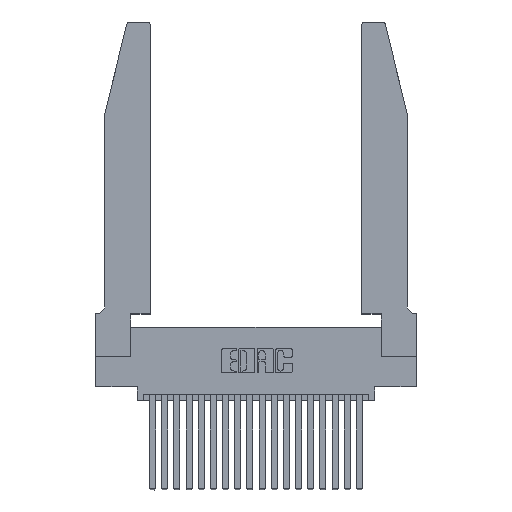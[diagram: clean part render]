
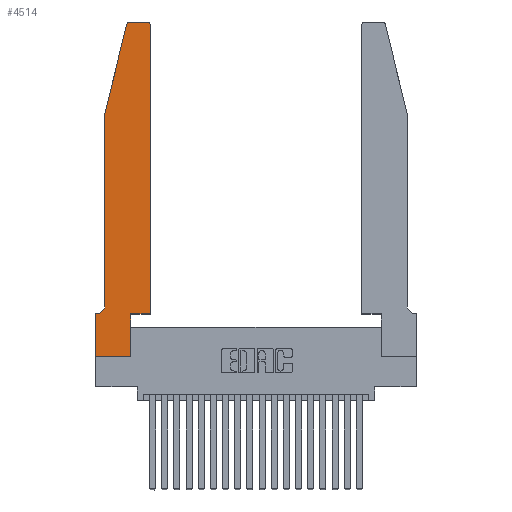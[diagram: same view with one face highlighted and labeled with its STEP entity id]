
A CAD part, top view. The second image highlights one B-rep face of the part: STEP entity #4514.
In plain terms, the highlighted planar face has unit normal (0, 0, 1).
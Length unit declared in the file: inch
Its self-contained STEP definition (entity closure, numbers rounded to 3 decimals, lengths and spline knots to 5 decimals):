
#236 = LINE ( 'NONE', #11558, #2390 ) ;
#587 = CARTESIAN_POINT ( 'NONE',  ( 0., 0., 0.37 ) ) ;
#653 = EDGE_CURVE ( 'NONE', #8122, #20150, #13571, .T. ) ;
#1013 = EDGE_CURVE ( 'NONE', #18267, #7652, #19644, .T. ) ;
#1073 = EDGE_CURVE ( 'NONE', #20150, #13080, #3122, .T. ) ;
#1366 = CIRCLE ( 'NONE', #17753, 0.03 ) ;
#1527 = DIRECTION ( 'NONE',  ( -1., 0., 0. ) ) ;
#1559 = DIRECTION ( 'NONE',  ( 1., 0., 0. ) ) ;
#1614 = VECTOR ( 'NONE', #1559, 39.37008 ) ;
#2044 = VECTOR ( 'NONE', #3336, 39.37008 ) ;
#2202 = AXIS2_PLACEMENT_3D ( 'NONE', #3374, #5071, #1527 ) ;
#2240 = CARTESIAN_POINT ( 'NONE',  ( 0., 0., 0.37 ) ) ;
#2390 = VECTOR ( 'NONE', #21987, 39.37008 ) ;
#2426 = LINE ( 'NONE', #10094, #1614 ) ;
#3022 = VERTEX_POINT ( 'NONE', #13504 ) ;
#3122 = LINE ( 'NONE', #21742, #2044 ) ;
#3255 = CARTESIAN_POINT ( 'NONE',  ( 0.4505, 0.35, 0.37 ) ) ;
#3336 = DIRECTION ( 'NONE',  ( -1., 0., 0. ) ) ;
#3374 = CARTESIAN_POINT ( 'NONE',  ( 0.0055, 0.42, 0.37 ) ) ;
#3446 = LINE ( 'NONE', #11900, #7200 ) ;
#3492 = LINE ( 'NONE', #2240, #19467 ) ;
#3637 = DIRECTION ( 'NONE',  ( 0., 0., 1. ) ) ;
#4107 = VERTEX_POINT ( 'NONE', #19464 ) ;
#4514 = ADVANCED_FACE ( 'NONE', ( #21670 ), #16902, .T. ) ;
#4571 = VERTEX_POINT ( 'NONE', #12188 ) ;
#4680 = DIRECTION ( 'NONE',  ( 1., 0., 0. ) ) ;
#4746 = CARTESIAN_POINT ( 'NONE',  ( 0.2605, 2.75, 0.37 ) ) ;
#5071 = DIRECTION ( 'NONE',  ( 0., 0., -1. ) ) ;
#5425 = DIRECTION ( 'NONE',  ( 1., 0., 0. ) ) ;
#5772 = VERTEX_POINT ( 'NONE', #10295 ) ;
#5898 = EDGE_CURVE ( 'NONE', #4107, #17096, #2426, .T. ) ;
#6042 = ORIENTED_EDGE ( 'NONE', *, *, #5898, .T. ) ;
#6260 = ORIENTED_EDGE ( 'NONE', *, *, #10911, .T. ) ;
#6274 = ORIENTED_EDGE ( 'NONE', *, *, #12861, .T. ) ;
#6558 = EDGE_CURVE ( 'NONE', #7302, #3022, #3446, .T. ) ;
#6589 = CARTESIAN_POINT ( 'NONE',  ( 0., 0.35, 0.37 ) ) ;
#7200 = VECTOR ( 'NONE', #20245, 39.37008 ) ;
#7202 = DIRECTION ( 'NONE',  ( 0., 0., 1. ) ) ;
#7302 = VERTEX_POINT ( 'NONE', #10898 ) ;
#7652 = VERTEX_POINT ( 'NONE', #21479 ) ;
#8122 = VERTEX_POINT ( 'NONE', #13676 ) ;
#8804 = CARTESIAN_POINT ( 'NONE',  ( 0.284, 2.72, 0.37 ) ) ;
#8990 = VECTOR ( 'NONE', #12801, 39.37008 ) ;
#10047 = EDGE_CURVE ( 'NONE', #4571, #5772, #3492, .T. ) ;
#10094 = CARTESIAN_POINT ( 'NONE',  ( 0.4505, 0.35, 0.37 ) ) ;
#10151 = CIRCLE ( 'NONE', #21735, 0.03 ) ;
#10295 = CARTESIAN_POINT ( 'NONE',  ( 0.2865, 0., 0.37 ) ) ;
#10708 = EDGE_LOOP ( 'NONE', ( #12510, #18027, #18974, #6260, #20082, #13953, #18576, #19677, #19640, #6042, #6274, #15577 ) ) ;
#10898 = CARTESIAN_POINT ( 'NONE',  ( 0.25487, 2.72718, 0.37 ) ) ;
#10911 = EDGE_CURVE ( 'NONE', #3022, #8122, #236, .T. ) ;
#10921 = DIRECTION ( 'NONE',  ( 1., 0., 0. ) ) ;
#11416 = EDGE_CURVE ( 'NONE', #7652, #7302, #10151, .T. ) ;
#11558 = CARTESIAN_POINT ( 'NONE',  ( 0.0755, 2., 0.37 ) ) ;
#11900 = CARTESIAN_POINT ( 'NONE',  ( 0.0755, 2., 0.37 ) ) ;
#12188 = CARTESIAN_POINT ( 'NONE',  ( 0., 0., 0.37 ) ) ;
#12228 = LINE ( 'NONE', #587, #17996 ) ;
#12309 = CARTESIAN_POINT ( 'NONE',  ( 0.4205, 2.72, 0.37 ) ) ;
#12510 = ORIENTED_EDGE ( 'NONE', *, *, #1013, .T. ) ;
#12565 = DIRECTION ( 'NONE',  ( 0., -1., 0. ) ) ;
#12801 = DIRECTION ( 'NONE',  ( 0., 1., 0. ) ) ;
#12861 = EDGE_CURVE ( 'NONE', #17096, #16095, #19310, .T. ) ;
#13064 = LINE ( 'NONE', #16942, #16998 ) ;
#13080 = VERTEX_POINT ( 'NONE', #18156 ) ;
#13114 = DIRECTION ( 'NONE',  ( 0., 1., 0. ) ) ;
#13446 = DIRECTION ( 'NONE',  ( 0., 0., 1. ) ) ;
#13504 = CARTESIAN_POINT ( 'NONE',  ( 0.0755, 2., 0.37 ) ) ;
#13571 = CIRCLE ( 'NONE', #2202, 0.07 ) ;
#13676 = CARTESIAN_POINT ( 'NONE',  ( 0.0755, 0.42, 0.37 ) ) ;
#13953 = ORIENTED_EDGE ( 'NONE', *, *, #1073, .T. ) ;
#14869 = VECTOR ( 'NONE', #19957, 39.37008 ) ;
#15368 = EDGE_CURVE ( 'NONE', #16095, #18267, #1366, .T. ) ;
#15422 = CARTESIAN_POINT ( 'NONE',  ( 0.0055, 0.35, 0.37 ) ) ;
#15577 = ORIENTED_EDGE ( 'NONE', *, *, #15368, .T. ) ;
#15705 = CARTESIAN_POINT ( 'NONE',  ( 0.4505, 2.72, 0.37 ) ) ;
#16095 = VERTEX_POINT ( 'NONE', #15705 ) ;
#16902 = PLANE ( 'NONE',  #21214 ) ;
#16942 = CARTESIAN_POINT ( 'NONE',  ( 0.2865, 0.35, 0.37 ) ) ;
#16998 = VECTOR ( 'NONE', #13114, 39.37008 ) ;
#17096 = VERTEX_POINT ( 'NONE', #3255 ) ;
#17134 = EDGE_CURVE ( 'NONE', #5772, #4107, #13064, .T. ) ;
#17252 = CARTESIAN_POINT ( 'NONE',  ( 0.4205, 2.75, 0.37 ) ) ;
#17753 = AXIS2_PLACEMENT_3D ( 'NONE', #12309, #7202, #20804 ) ;
#17996 = VECTOR ( 'NONE', #12565, 39.37008 ) ;
#18027 = ORIENTED_EDGE ( 'NONE', *, *, #11416, .T. ) ;
#18156 = CARTESIAN_POINT ( 'NONE',  ( 0., 0.35, 0.37 ) ) ;
#18267 = VERTEX_POINT ( 'NONE', #17252 ) ;
#18504 = EDGE_CURVE ( 'NONE', #13080, #4571, #12228, .T. ) ;
#18576 = ORIENTED_EDGE ( 'NONE', *, *, #18504, .T. ) ;
#18974 = ORIENTED_EDGE ( 'NONE', *, *, #6558, .T. ) ;
#19310 = LINE ( 'NONE', #19743, #8990 ) ;
#19464 = CARTESIAN_POINT ( 'NONE',  ( 0.2865, 0.35, 0.37 ) ) ;
#19467 = VECTOR ( 'NONE', #10921, 39.37008 ) ;
#19640 = ORIENTED_EDGE ( 'NONE', *, *, #17134, .T. ) ;
#19644 = LINE ( 'NONE', #4746, #14869 ) ;
#19677 = ORIENTED_EDGE ( 'NONE', *, *, #10047, .T. ) ;
#19743 = CARTESIAN_POINT ( 'NONE',  ( 0.4505, 0.35, 0.37 ) ) ;
#19957 = DIRECTION ( 'NONE',  ( -1., 0., 0. ) ) ;
#20082 = ORIENTED_EDGE ( 'NONE', *, *, #653, .T. ) ;
#20150 = VERTEX_POINT ( 'NONE', #15422 ) ;
#20245 = DIRECTION ( 'NONE',  ( -0.239, -0.971, 0. ) ) ;
#20804 = DIRECTION ( 'NONE',  ( 1., 0., 0. ) ) ;
#21214 = AXIS2_PLACEMENT_3D ( 'NONE', #6589, #13446, #4680 ) ;
#21479 = CARTESIAN_POINT ( 'NONE',  ( 0.284, 2.75, 0.37 ) ) ;
#21670 = FACE_OUTER_BOUND ( 'NONE', #10708, .T. ) ;
#21735 = AXIS2_PLACEMENT_3D ( 'NONE', #8804, #3637, #5425 ) ;
#21742 = CARTESIAN_POINT ( 'NONE',  ( 0.0755, 0.35, 0.37 ) ) ;
#21987 = DIRECTION ( 'NONE',  ( 0., -1., 0. ) ) ;
